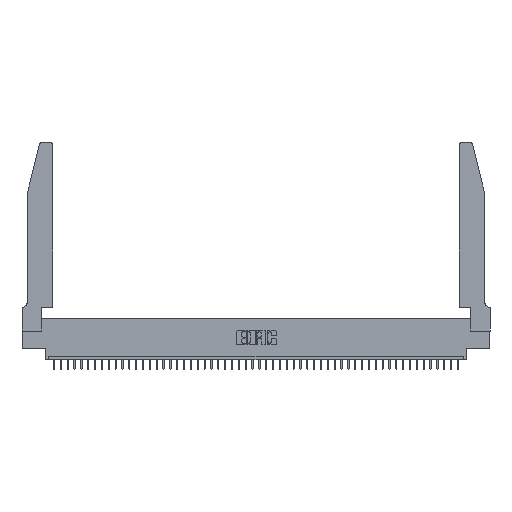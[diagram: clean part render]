
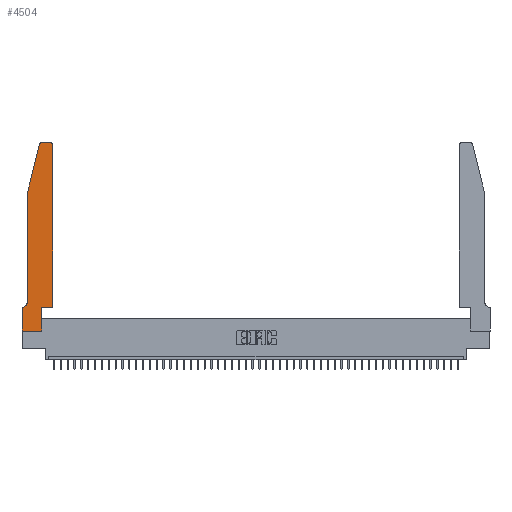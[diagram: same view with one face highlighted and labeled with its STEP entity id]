
A CAD part, top view. The second image highlights one B-rep face of the part: STEP entity #4504.
In plain terms, the highlighted planar face has unit normal (0, 0, 1).
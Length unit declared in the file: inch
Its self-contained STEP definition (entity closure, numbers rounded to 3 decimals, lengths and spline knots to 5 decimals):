
#32 = ORIENTED_EDGE ( 'NONE', *, *, #1556, .T. ) ;
#840 = LINE ( 'NONE', #8540, #47281 ) ;
#1267 = EDGE_CURVE ( 'NONE', #45213, #27555, #1601, .T. ) ;
#1556 = EDGE_CURVE ( 'NONE', #47363, #43411, #1665, .T. ) ;
#1601 = LINE ( 'NONE', #5444, #27034 ) ;
#1665 = CIRCLE ( 'NONE', #43247, 0.03 ) ;
#2209 = ORIENTED_EDGE ( 'NONE', *, *, #34622, .T. ) ;
#2232 = LINE ( 'NONE', #43233, #42904 ) ;
#2439 = VECTOR ( 'NONE', #6994, 39.37008 ) ;
#3289 = FACE_OUTER_BOUND ( 'NONE', #37778, .T. ) ;
#3798 = DIRECTION ( 'NONE',  ( 1., 0., 0. ) ) ;
#4504 = ADVANCED_FACE ( 'NONE', ( #3289 ), #17990, .T. ) ;
#5262 = CARTESIAN_POINT ( 'NONE',  ( 0.0755, 2., 0.37 ) ) ;
#5444 = CARTESIAN_POINT ( 'NONE',  ( 0.0755, 0.35, 0.37 ) ) ;
#5507 = CARTESIAN_POINT ( 'NONE',  ( 0.25487, 2.72718, 0.37 ) ) ;
#5614 = LINE ( 'NONE', #25321, #47213 ) ;
#6310 = ORIENTED_EDGE ( 'NONE', *, *, #13568, .T. ) ;
#6976 = CARTESIAN_POINT ( 'NONE',  ( 0., 0., 0.37 ) ) ;
#6994 = DIRECTION ( 'NONE',  ( -1., 0., 0. ) ) ;
#7329 = DIRECTION ( 'NONE',  ( 0., 0., 1. ) ) ;
#8540 = CARTESIAN_POINT ( 'NONE',  ( 0.4505, 0.35, 0.37 ) ) ;
#9147 = DIRECTION ( 'NONE',  ( 1., 0., 0. ) ) ;
#9792 = DIRECTION ( 'NONE',  ( 0., 0., 1. ) ) ;
#11414 = EDGE_CURVE ( 'NONE', #38718, #47363, #2232, .T. ) ;
#11546 = EDGE_CURVE ( 'NONE', #15696, #30474, #16384, .T. ) ;
#12039 = AXIS2_PLACEMENT_3D ( 'NONE', #34326, #15701, #45187 ) ;
#12545 = VECTOR ( 'NONE', #25089, 39.37008 ) ;
#13106 = ORIENTED_EDGE ( 'NONE', *, *, #11414, .T. ) ;
#13326 = DIRECTION ( 'NONE',  ( 1., 0., 0. ) ) ;
#13547 = CARTESIAN_POINT ( 'NONE',  ( 0.0055, 0.35, 0.37 ) ) ;
#13568 = EDGE_CURVE ( 'NONE', #27947, #33998, #31083, .T. ) ;
#14256 = CARTESIAN_POINT ( 'NONE',  ( 0., 0.35, 0.37 ) ) ;
#14355 = VECTOR ( 'NONE', #9147, 39.37008 ) ;
#15116 = CIRCLE ( 'NONE', #12039, 0.07 ) ;
#15122 = CARTESIAN_POINT ( 'NONE',  ( 0.4205, 2.75, 0.37 ) ) ;
#15696 = VERTEX_POINT ( 'NONE', #6976 ) ;
#15701 = DIRECTION ( 'NONE',  ( 0., 0., -1. ) ) ;
#16384 = LINE ( 'NONE', #42221, #14355 ) ;
#16696 = EDGE_CURVE ( 'NONE', #33998, #31658, #31225, .T. ) ;
#16928 = DIRECTION ( 'NONE',  ( 0., 1., 0. ) ) ;
#17227 = EDGE_CURVE ( 'NONE', #39187, #27947, #22605, .T. ) ;
#17513 = CARTESIAN_POINT ( 'NONE',  ( 0., 0.35, 0.37 ) ) ;
#17990 = PLANE ( 'NONE',  #44220 ) ;
#18095 = LINE ( 'NONE', #29435, #2439 ) ;
#18245 = EDGE_CURVE ( 'NONE', #30474, #45823, #30695, .T. ) ;
#18261 = DIRECTION ( 'NONE',  ( 0., 0., 1. ) ) ;
#19463 = VECTOR ( 'NONE', #45429, 39.37008 ) ;
#22605 = CIRCLE ( 'NONE', #24120, 0.03 ) ;
#23830 = ORIENTED_EDGE ( 'NONE', *, *, #31362, .T. ) ;
#23908 = ORIENTED_EDGE ( 'NONE', *, *, #1267, .T. ) ;
#24120 = AXIS2_PLACEMENT_3D ( 'NONE', #40949, #18261, #3798 ) ;
#24621 = ORIENTED_EDGE ( 'NONE', *, *, #16696, .T. ) ;
#25089 = DIRECTION ( 'NONE',  ( 0., -1., 0. ) ) ;
#25321 = CARTESIAN_POINT ( 'NONE',  ( 0., 0., 0.37 ) ) ;
#26028 = CARTESIAN_POINT ( 'NONE',  ( 0.0755, 0.42, 0.37 ) ) ;
#26272 = CARTESIAN_POINT ( 'NONE',  ( 0.4505, 0.35, 0.37 ) ) ;
#26825 = CARTESIAN_POINT ( 'NONE',  ( 0.2865, 0.35, 0.37 ) ) ;
#27034 = VECTOR ( 'NONE', #35133, 39.37008 ) ;
#27555 = VERTEX_POINT ( 'NONE', #14256 ) ;
#27947 = VERTEX_POINT ( 'NONE', #5507 ) ;
#28946 = EDGE_CURVE ( 'NONE', #27555, #15696, #5614, .T. ) ;
#29435 = CARTESIAN_POINT ( 'NONE',  ( 0.2605, 2.75, 0.37 ) ) ;
#30474 = VERTEX_POINT ( 'NONE', #41789 ) ;
#30695 = LINE ( 'NONE', #26825, #19463 ) ;
#31083 = LINE ( 'NONE', #5262, #32722 ) ;
#31225 = LINE ( 'NONE', #45959, #12545 ) ;
#31362 = EDGE_CURVE ( 'NONE', #45823, #38718, #840, .T. ) ;
#31658 = VERTEX_POINT ( 'NONE', #26028 ) ;
#32254 = DIRECTION ( 'NONE',  ( 1., 0., 0. ) ) ;
#32722 = VECTOR ( 'NONE', #46506, 39.37008 ) ;
#33998 = VERTEX_POINT ( 'NONE', #37525 ) ;
#34326 = CARTESIAN_POINT ( 'NONE',  ( 0.0055, 0.42, 0.37 ) ) ;
#34622 = EDGE_CURVE ( 'NONE', #31658, #45213, #15116, .T. ) ;
#34691 = CARTESIAN_POINT ( 'NONE',  ( 0.2865, 0.35, 0.37 ) ) ;
#34847 = DIRECTION ( 'NONE',  ( 0., -1., 0. ) ) ;
#35133 = DIRECTION ( 'NONE',  ( -1., 0., 0. ) ) ;
#35855 = ORIENTED_EDGE ( 'NONE', *, *, #18245, .T. ) ;
#36884 = CARTESIAN_POINT ( 'NONE',  ( 0.4505, 2.72, 0.37 ) ) ;
#37525 = CARTESIAN_POINT ( 'NONE',  ( 0.0755, 2., 0.37 ) ) ;
#37778 = EDGE_LOOP ( 'NONE', ( #47131, #44708, #6310, #24621, #2209, #23908, #44992, #39772, #35855, #23830, #13106, #32 ) ) ;
#38718 = VERTEX_POINT ( 'NONE', #26272 ) ;
#39187 = VERTEX_POINT ( 'NONE', #43255 ) ;
#39772 = ORIENTED_EDGE ( 'NONE', *, *, #11546, .T. ) ;
#40949 = CARTESIAN_POINT ( 'NONE',  ( 0.284, 2.72, 0.37 ) ) ;
#41358 = CARTESIAN_POINT ( 'NONE',  ( 0.4205, 2.72, 0.37 ) ) ;
#41789 = CARTESIAN_POINT ( 'NONE',  ( 0.2865, 0., 0.37 ) ) ;
#42221 = CARTESIAN_POINT ( 'NONE',  ( 0., 0., 0.37 ) ) ;
#42904 = VECTOR ( 'NONE', #16928, 39.37008 ) ;
#43233 = CARTESIAN_POINT ( 'NONE',  ( 0.4505, 0.35, 0.37 ) ) ;
#43247 = AXIS2_PLACEMENT_3D ( 'NONE', #41358, #7329, #44745 ) ;
#43255 = CARTESIAN_POINT ( 'NONE',  ( 0.284, 2.75, 0.37 ) ) ;
#43411 = VERTEX_POINT ( 'NONE', #15122 ) ;
#44220 = AXIS2_PLACEMENT_3D ( 'NONE', #17513, #9792, #32254 ) ;
#44708 = ORIENTED_EDGE ( 'NONE', *, *, #17227, .T. ) ;
#44745 = DIRECTION ( 'NONE',  ( 1., 0., 0. ) ) ;
#44992 = ORIENTED_EDGE ( 'NONE', *, *, #28946, .T. ) ;
#45187 = DIRECTION ( 'NONE',  ( -1., 0., 0. ) ) ;
#45213 = VERTEX_POINT ( 'NONE', #13547 ) ;
#45429 = DIRECTION ( 'NONE',  ( 0., 1., 0. ) ) ;
#45823 = VERTEX_POINT ( 'NONE', #34691 ) ;
#45959 = CARTESIAN_POINT ( 'NONE',  ( 0.0755, 2., 0.37 ) ) ;
#46506 = DIRECTION ( 'NONE',  ( -0.239, -0.971, 0. ) ) ;
#46920 = EDGE_CURVE ( 'NONE', #43411, #39187, #18095, .T. ) ;
#47131 = ORIENTED_EDGE ( 'NONE', *, *, #46920, .T. ) ;
#47213 = VECTOR ( 'NONE', #34847, 39.37008 ) ;
#47281 = VECTOR ( 'NONE', #13326, 39.37008 ) ;
#47363 = VERTEX_POINT ( 'NONE', #36884 ) ;
